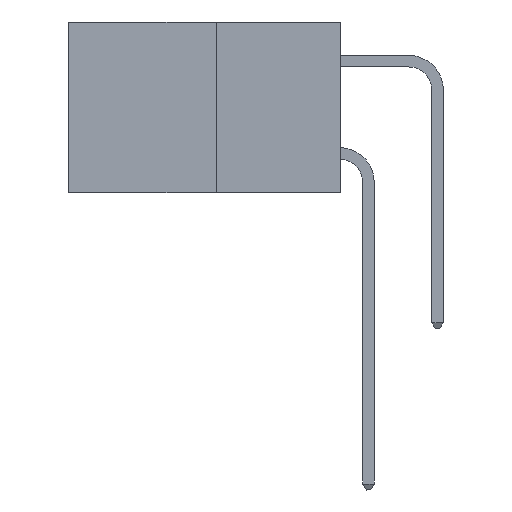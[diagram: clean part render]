
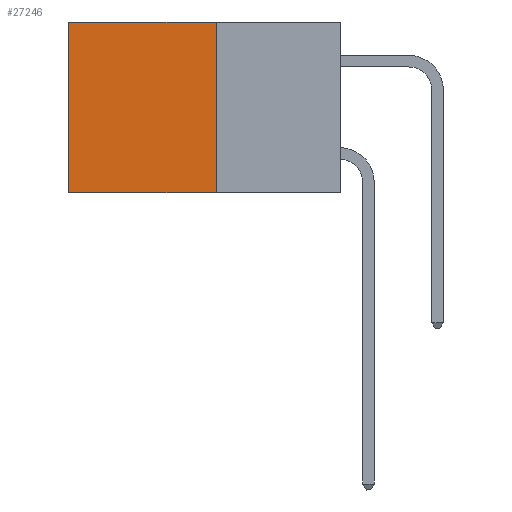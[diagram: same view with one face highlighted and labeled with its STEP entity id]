
A CAD part, left-side view. The second image highlights one B-rep face of the part: STEP entity #27246.
In plain terms, the highlighted planar face has unit normal (-1, 0, 0).
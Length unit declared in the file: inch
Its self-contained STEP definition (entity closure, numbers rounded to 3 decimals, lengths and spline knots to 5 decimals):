
#2104 = CARTESIAN_POINT ( 'NONE',  ( 0.277, 0.59, -0.37 ) ) ;
#2422 = DIRECTION ( 'NONE',  ( 0., 1., 0. ) ) ;
#4091 = DIRECTION ( 'NONE',  ( 0., 1., 0. ) ) ;
#5059 = VECTOR ( 'NONE', #4091, 39.37008 ) ;
#8907 = CARTESIAN_POINT ( 'NONE',  ( 0.277, 0.27, -0.37 ) ) ;
#9583 = AXIS2_PLACEMENT_3D ( 'NONE', #27434, #10169, #25386 ) ;
#10169 = DIRECTION ( 'NONE',  ( 1., 0., 0. ) ) ;
#10202 = LINE ( 'NONE', #10604, #15396 ) ;
#10347 = VERTEX_POINT ( 'NONE', #22593 ) ;
#10582 = CARTESIAN_POINT ( 'NONE',  ( 0.277, 0.27, 0. ) ) ;
#10604 = CARTESIAN_POINT ( 'NONE',  ( 0.277, 0.27, -0.37 ) ) ;
#10826 = LINE ( 'NONE', #23682, #5059 ) ;
#10828 = VECTOR ( 'NONE', #15253, 39.37008 ) ;
#11658 = EDGE_CURVE ( 'NONE', #16250, #13997, #27536, .T. ) ;
#13521 = ORIENTED_EDGE ( 'NONE', *, *, #17440, .F. ) ;
#13997 = VERTEX_POINT ( 'NONE', #25077 ) ;
#15253 = DIRECTION ( 'NONE',  ( 0., 0., -1. ) ) ;
#15396 = VECTOR ( 'NONE', #27945, 39.37008 ) ;
#16250 = VERTEX_POINT ( 'NONE', #16495 ) ;
#16495 = CARTESIAN_POINT ( 'NONE',  ( 0.277, 0.27, -0.37 ) ) ;
#17440 = EDGE_CURVE ( 'NONE', #18060, #16250, #10202, .T. ) ;
#18029 = ORIENTED_EDGE ( 'NONE', *, *, #21649, .T. ) ;
#18060 = VERTEX_POINT ( 'NONE', #10582 ) ;
#18629 = ORIENTED_EDGE ( 'NONE', *, *, #11658, .F. ) ;
#19305 = ORIENTED_EDGE ( 'NONE', *, *, #19491, .T. ) ;
#19491 = EDGE_CURVE ( 'NONE', #10347, #13997, #28111, .T. ) ;
#21152 = VECTOR ( 'NONE', #2422, 39.37008 ) ;
#21649 = EDGE_CURVE ( 'NONE', #18060, #10347, #10826, .T. ) ;
#22444 = EDGE_LOOP ( 'NONE', ( #19305, #18629, #13521, #18029 ) ) ;
#22593 = CARTESIAN_POINT ( 'NONE',  ( 0.277, 0.59, 0. ) ) ;
#23211 = PLANE ( 'NONE',  #9583 ) ;
#23682 = CARTESIAN_POINT ( 'NONE',  ( 0.277, 0.27, 0. ) ) ;
#25077 = CARTESIAN_POINT ( 'NONE',  ( 0.277, 0.59, -0.37 ) ) ;
#25386 = DIRECTION ( 'NONE',  ( 0., 0., -1. ) ) ;
#25856 = FACE_OUTER_BOUND ( 'NONE', #22444, .T. ) ;
#27246 = ADVANCED_FACE ( 'NONE', ( #25856 ), #23211, .F. ) ;
#27434 = CARTESIAN_POINT ( 'NONE',  ( 0.277, 0.27, -0.37 ) ) ;
#27536 = LINE ( 'NONE', #8907, #21152 ) ;
#27945 = DIRECTION ( 'NONE',  ( 0., 0., -1. ) ) ;
#28111 = LINE ( 'NONE', #2104, #10828 ) ;
